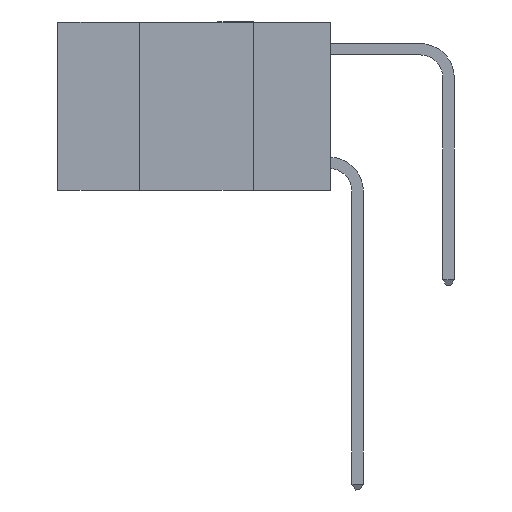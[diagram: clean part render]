
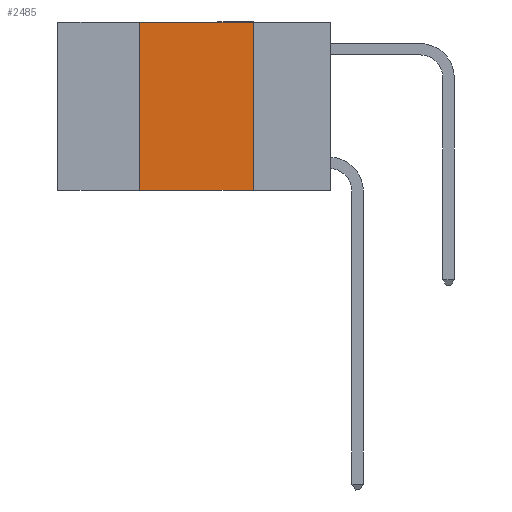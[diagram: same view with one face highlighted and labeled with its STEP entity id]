
A CAD part, left-side view. The second image highlights one B-rep face of the part: STEP entity #2485.
In plain terms, the highlighted planar face has unit normal (-1, 0, 0).
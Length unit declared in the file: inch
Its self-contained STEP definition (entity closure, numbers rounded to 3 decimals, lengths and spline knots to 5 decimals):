
#513 = VECTOR ( 'NONE', #4120, 39.37008 ) ;
#686 = FACE_OUTER_BOUND ( 'NONE', #7656, .T. ) ;
#1226 = EDGE_CURVE ( 'NONE', #1750, #8200, #7623, .T. ) ;
#1420 = VERTEX_POINT ( 'NONE', #6279 ) ;
#1528 = ORIENTED_EDGE ( 'NONE', *, *, #1226, .F. ) ;
#1750 = VERTEX_POINT ( 'NONE', #5590 ) ;
#2485 = ADVANCED_FACE ( 'NONE', ( #686 ), #5437, .F. ) ;
#2564 = ORIENTED_EDGE ( 'NONE', *, *, #5510, .F. ) ;
#2749 = DIRECTION ( 'NONE',  ( 0., 0., 1. ) ) ;
#3070 = EDGE_CURVE ( 'NONE', #1420, #6853, #7184, .T. ) ;
#3082 = ORIENTED_EDGE ( 'NONE', *, *, #3070, .F. ) ;
#3120 = CARTESIAN_POINT ( 'NONE',  ( 0., 0.17, -0.37 ) ) ;
#4040 = CARTESIAN_POINT ( 'NONE',  ( 0., 0.42, 0. ) ) ;
#4063 = LINE ( 'NONE', #8993, #10446 ) ;
#4104 = DIRECTION ( 'NONE',  ( 0., -1., 0. ) ) ;
#4120 = DIRECTION ( 'NONE',  ( 0., 0., -1. ) ) ;
#4560 = LINE ( 'NONE', #9099, #6006 ) ;
#5375 = DIRECTION ( 'NONE',  ( 0., 0., -1. ) ) ;
#5393 = DIRECTION ( 'NONE',  ( 1., 0., 0. ) ) ;
#5437 = PLANE ( 'NONE',  #9420 ) ;
#5510 = EDGE_CURVE ( 'NONE', #8200, #1420, #4560, .T. ) ;
#5557 = CARTESIAN_POINT ( 'NONE',  ( 0., 0.6, 0. ) ) ;
#5590 = CARTESIAN_POINT ( 'NONE',  ( 0., 0.42, -0.37 ) ) ;
#6006 = VECTOR ( 'NONE', #4104, 39.37008 ) ;
#6279 = CARTESIAN_POINT ( 'NONE',  ( 0., 0.17, 0. ) ) ;
#6446 = DIRECTION ( 'NONE',  ( 0., -1., 0. ) ) ;
#6853 = VERTEX_POINT ( 'NONE', #3120 ) ;
#7184 = LINE ( 'NONE', #10748, #513 ) ;
#7623 = LINE ( 'NONE', #4040, #9857 ) ;
#7656 = EDGE_LOOP ( 'NONE', ( #3082, #2564, #1528, #9576 ) ) ;
#8200 = VERTEX_POINT ( 'NONE', #8536 ) ;
#8536 = CARTESIAN_POINT ( 'NONE',  ( 0., 0.42, 0. ) ) ;
#8993 = CARTESIAN_POINT ( 'NONE',  ( 0., 0.6, -0.37 ) ) ;
#9099 = CARTESIAN_POINT ( 'NONE',  ( 0., 0.6, 0. ) ) ;
#9420 = AXIS2_PLACEMENT_3D ( 'NONE', #5557, #5393, #5375 ) ;
#9576 = ORIENTED_EDGE ( 'NONE', *, *, #11014, .T. ) ;
#9857 = VECTOR ( 'NONE', #2749, 39.37008 ) ;
#10446 = VECTOR ( 'NONE', #6446, 39.37008 ) ;
#10748 = CARTESIAN_POINT ( 'NONE',  ( 0., 0.17, 0. ) ) ;
#11014 = EDGE_CURVE ( 'NONE', #1750, #6853, #4063, .T. ) ;
